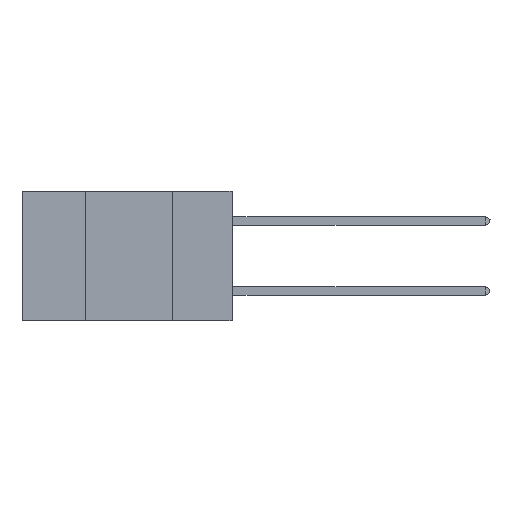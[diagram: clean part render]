
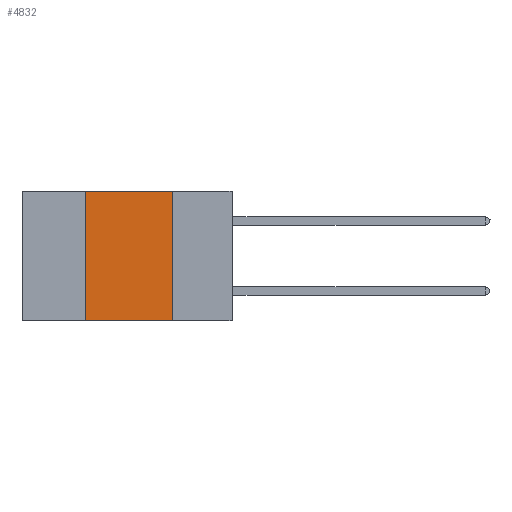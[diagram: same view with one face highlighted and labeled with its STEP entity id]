
A CAD part, left-side view. The second image highlights one B-rep face of the part: STEP entity #4832.
In plain terms, the highlighted planar face has unit normal (-1, 0, 0).
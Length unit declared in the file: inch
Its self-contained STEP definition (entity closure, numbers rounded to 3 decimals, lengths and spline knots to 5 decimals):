
#852 = PLANE ( 'NONE',  #20376 ) ;
#3065 = LINE ( 'NONE', #10376, #18286 ) ;
#4338 = CARTESIAN_POINT ( 'NONE',  ( 0., 0.17, 0. ) ) ;
#4832 = ADVANCED_FACE ( 'NONE', ( #17188 ), #852, .F. ) ;
#5223 = VERTEX_POINT ( 'NONE', #8371 ) ;
#5299 = CARTESIAN_POINT ( 'NONE',  ( 0., 0.42, -0.37 ) ) ;
#5460 = LINE ( 'NONE', #12754, #8713 ) ;
#6502 = DIRECTION ( 'NONE',  ( 0., 0., -1. ) ) ;
#8371 = CARTESIAN_POINT ( 'NONE',  ( 0., 0.42, 0. ) ) ;
#8713 = VECTOR ( 'NONE', #19995, 39.37008 ) ;
#9568 = CARTESIAN_POINT ( 'NONE',  ( 0., 0.6, -0.37 ) ) ;
#9866 = ORIENTED_EDGE ( 'NONE', *, *, #16931, .F. ) ;
#10376 = CARTESIAN_POINT ( 'NONE',  ( 0., 0.17, 0. ) ) ;
#10498 = EDGE_CURVE ( 'NONE', #20263, #11172, #19905, .T. ) ;
#10628 = ORIENTED_EDGE ( 'NONE', *, *, #14604, .F. ) ;
#11172 = VERTEX_POINT ( 'NONE', #22747 ) ;
#11405 = EDGE_LOOP ( 'NONE', ( #9866, #19346, #10628, #20394 ) ) ;
#12754 = CARTESIAN_POINT ( 'NONE',  ( 0., 0.42, 0. ) ) ;
#13772 = VECTOR ( 'NONE', #15803, 39.37008 ) ;
#14604 = EDGE_CURVE ( 'NONE', #20263, #5223, #5460, .T. ) ;
#15415 = CARTESIAN_POINT ( 'NONE',  ( 0., 0.6, 0. ) ) ;
#15803 = DIRECTION ( 'NONE',  ( 0., -1., 0. ) ) ;
#16687 = DIRECTION ( 'NONE',  ( 0., -1., 0. ) ) ;
#16931 = EDGE_CURVE ( 'NONE', #23208, #11172, #3065, .T. ) ;
#16975 = VECTOR ( 'NONE', #16687, 39.37008 ) ;
#17188 = FACE_OUTER_BOUND ( 'NONE', #11405, .T. ) ;
#18286 = VECTOR ( 'NONE', #22218, 39.37008 ) ;
#19346 = ORIENTED_EDGE ( 'NONE', *, *, #19939, .F. ) ;
#19905 = LINE ( 'NONE', #9568, #16975 ) ;
#19939 = EDGE_CURVE ( 'NONE', #5223, #23208, #23215, .T. ) ;
#19995 = DIRECTION ( 'NONE',  ( 0., 0., 1. ) ) ;
#20263 = VERTEX_POINT ( 'NONE', #5299 ) ;
#20376 = AXIS2_PLACEMENT_3D ( 'NONE', #15415, #20912, #6502 ) ;
#20394 = ORIENTED_EDGE ( 'NONE', *, *, #10498, .T. ) ;
#20912 = DIRECTION ( 'NONE',  ( 1., 0., 0. ) ) ;
#22218 = DIRECTION ( 'NONE',  ( 0., 0., -1. ) ) ;
#22747 = CARTESIAN_POINT ( 'NONE',  ( 0., 0.17, -0.37 ) ) ;
#23102 = CARTESIAN_POINT ( 'NONE',  ( 0., 0.6, 0. ) ) ;
#23208 = VERTEX_POINT ( 'NONE', #4338 ) ;
#23215 = LINE ( 'NONE', #23102, #13772 ) ;
